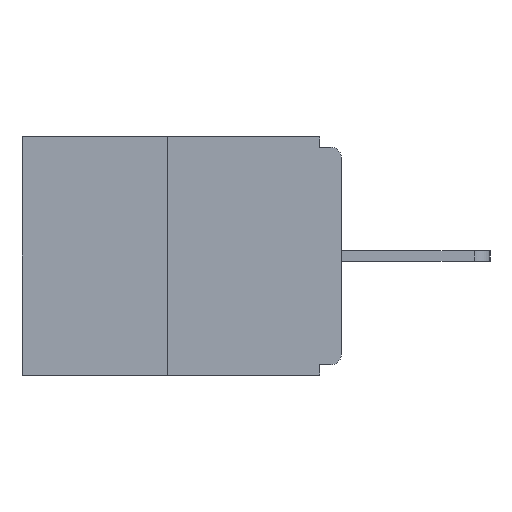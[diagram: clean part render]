
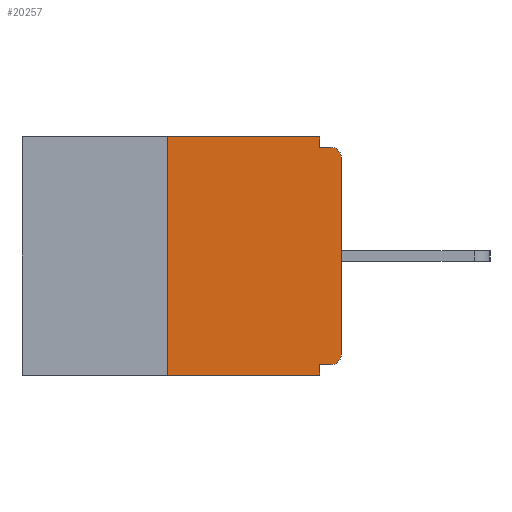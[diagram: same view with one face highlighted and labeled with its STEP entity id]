
A CAD part, left-side view. The second image highlights one B-rep face of the part: STEP entity #20257.
In plain terms, the highlighted planar face has unit normal (-1, 0, 0).
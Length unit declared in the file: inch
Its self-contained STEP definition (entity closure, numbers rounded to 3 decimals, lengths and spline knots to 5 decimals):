
#117 = VECTOR ( 'NONE', #4930, 39.37008 ) ;
#574 = DIRECTION ( 'NONE',  ( 0., -1., 0. ) ) ;
#755 = ORIENTED_EDGE ( 'NONE', *, *, #6911, .F. ) ;
#1035 = VECTOR ( 'NONE', #574, 39.37008 ) ;
#2110 = EDGE_CURVE ( 'NONE', #6179, #14480, #10528, .T. ) ;
#2219 = LINE ( 'NONE', #10563, #1035 ) ;
#2291 = VERTEX_POINT ( 'NONE', #3269 ) ;
#2664 = VERTEX_POINT ( 'NONE', #17698 ) ;
#2714 = CARTESIAN_POINT ( 'NONE',  ( 0., 0.031, 0. ) ) ;
#2983 = ORIENTED_EDGE ( 'NONE', *, *, #8985, .F. ) ;
#3269 = CARTESIAN_POINT ( 'NONE',  ( 0., 0.25, -0.343 ) ) ;
#3301 = ORIENTED_EDGE ( 'NONE', *, *, #9194, .T. ) ;
#3342 = CIRCLE ( 'NONE', #20670, 0.015 ) ;
#3399 = CARTESIAN_POINT ( 'NONE',  ( 0., 0., -0.328 ) ) ;
#3410 = CARTESIAN_POINT ( 'NONE',  ( 0., 0., -0.015 ) ) ;
#3615 = DIRECTION ( 'NONE',  ( 0., 0., 1. ) ) ;
#3663 = VERTEX_POINT ( 'NONE', #17175 ) ;
#3956 = ORIENTED_EDGE ( 'NONE', *, *, #13692, .F. ) ;
#4565 = VECTOR ( 'NONE', #20036, 39.37008 ) ;
#4846 = EDGE_CURVE ( 'NONE', #13878, #9414, #21352, .T. ) ;
#4930 = DIRECTION ( 'NONE',  ( 0., 0., -1. ) ) ;
#4979 = VECTOR ( 'NONE', #15206, 39.37008 ) ;
#5287 = ORIENTED_EDGE ( 'NONE', *, *, #14898, .F. ) ;
#6045 = AXIS2_PLACEMENT_3D ( 'NONE', #9595, #14525, #11502 ) ;
#6106 = VERTEX_POINT ( 'NONE', #14680 ) ;
#6179 = VERTEX_POINT ( 'NONE', #20354 ) ;
#6204 = DIRECTION ( 'NONE',  ( 0., 0., -1. ) ) ;
#6223 = FACE_OUTER_BOUND ( 'NONE', #15611, .T. ) ;
#6728 = LINE ( 'NONE', #12034, #15156 ) ;
#6911 = EDGE_CURVE ( 'NONE', #2664, #8474, #21631, .T. ) ;
#8474 = VERTEX_POINT ( 'NONE', #15916 ) ;
#8921 = CARTESIAN_POINT ( 'NONE',  ( 0., 0.031, -0.015 ) ) ;
#8985 = EDGE_CURVE ( 'NONE', #9414, #6106, #18573, .T. ) ;
#9194 = EDGE_CURVE ( 'NONE', #14480, #6106, #3342, .T. ) ;
#9414 = VERTEX_POINT ( 'NONE', #8921 ) ;
#9595 = CARTESIAN_POINT ( 'NONE',  ( 0., 0.015, -0.313 ) ) ;
#9598 = CIRCLE ( 'NONE', #6045, 0.015 ) ;
#10102 = VECTOR ( 'NONE', #16882, 39.37008 ) ;
#10528 = LINE ( 'NONE', #17203, #20855 ) ;
#10563 = CARTESIAN_POINT ( 'NONE',  ( 0., 0.46, 0. ) ) ;
#11502 = DIRECTION ( 'NONE',  ( 0., 0., -1. ) ) ;
#11679 = CARTESIAN_POINT ( 'NONE',  ( 0., 0., -0.03 ) ) ;
#12034 = CARTESIAN_POINT ( 'NONE',  ( 0., 0.25, 0. ) ) ;
#12941 = PLANE ( 'NONE',  #17561 ) ;
#13042 = EDGE_CURVE ( 'NONE', #2291, #8474, #14574, .T. ) ;
#13259 = CARTESIAN_POINT ( 'NONE',  ( 0., 0.46, -0.343 ) ) ;
#13692 = EDGE_CURVE ( 'NONE', #2291, #17548, #6728, .T. ) ;
#13878 = VERTEX_POINT ( 'NONE', #2714 ) ;
#14049 = ORIENTED_EDGE ( 'NONE', *, *, #20490, .F. ) ;
#14204 = CARTESIAN_POINT ( 'NONE',  ( 0., 0.015, -0.03 ) ) ;
#14217 = VECTOR ( 'NONE', #6204, 39.37008 ) ;
#14480 = VERTEX_POINT ( 'NONE', #11679 ) ;
#14525 = DIRECTION ( 'NONE',  ( -1., 0., 0. ) ) ;
#14574 = LINE ( 'NONE', #13259, #4565 ) ;
#14680 = CARTESIAN_POINT ( 'NONE',  ( 0., 0.015, -0.015 ) ) ;
#14898 = EDGE_CURVE ( 'NONE', #3663, #2664, #18562, .T. ) ;
#15146 = EDGE_CURVE ( 'NONE', #3663, #6179, #9598, .T. ) ;
#15156 = VECTOR ( 'NONE', #3615, 39.37008 ) ;
#15206 = DIRECTION ( 'NONE',  ( 0., 1., 0. ) ) ;
#15210 = DIRECTION ( 'NONE',  ( 0., 0., 1. ) ) ;
#15517 = ORIENTED_EDGE ( 'NONE', *, *, #4846, .F. ) ;
#15611 = EDGE_LOOP ( 'NONE', ( #14049, #3956, #17059, #755, #5287, #18171, #20974, #3301, #2983, #15517 ) ) ;
#15916 = CARTESIAN_POINT ( 'NONE',  ( 0., 0.031, -0.343 ) ) ;
#15958 = DIRECTION ( 'NONE',  ( -1., 0., 0. ) ) ;
#16303 = DIRECTION ( 'NONE',  ( 0., 0., -1. ) ) ;
#16882 = DIRECTION ( 'NONE',  ( 0., -1., 0. ) ) ;
#17059 = ORIENTED_EDGE ( 'NONE', *, *, #13042, .T. ) ;
#17175 = CARTESIAN_POINT ( 'NONE',  ( 0., 0.015, -0.328 ) ) ;
#17203 = CARTESIAN_POINT ( 'NONE',  ( 0., 0., 0. ) ) ;
#17548 = VERTEX_POINT ( 'NONE', #19046 ) ;
#17561 = AXIS2_PLACEMENT_3D ( 'NONE', #19721, #18052, #21806 ) ;
#17698 = CARTESIAN_POINT ( 'NONE',  ( 0., 0.031, -0.328 ) ) ;
#18052 = DIRECTION ( 'NONE',  ( 1., 0., 0. ) ) ;
#18171 = ORIENTED_EDGE ( 'NONE', *, *, #15146, .T. ) ;
#18470 = CARTESIAN_POINT ( 'NONE',  ( 0., 0.031, 0. ) ) ;
#18562 = LINE ( 'NONE', #3399, #4979 ) ;
#18573 = LINE ( 'NONE', #3410, #10102 ) ;
#19046 = CARTESIAN_POINT ( 'NONE',  ( 0., 0.25, 0. ) ) ;
#19721 = CARTESIAN_POINT ( 'NONE',  ( 0., 0.46, 0. ) ) ;
#20036 = DIRECTION ( 'NONE',  ( 0., -1., 0. ) ) ;
#20257 = ADVANCED_FACE ( 'NONE', ( #6223 ), #12941, .F. ) ;
#20354 = CARTESIAN_POINT ( 'NONE',  ( 0., 0., -0.313 ) ) ;
#20490 = EDGE_CURVE ( 'NONE', #17548, #13878, #2219, .T. ) ;
#20670 = AXIS2_PLACEMENT_3D ( 'NONE', #14204, #15958, #16303 ) ;
#20855 = VECTOR ( 'NONE', #15210, 39.37008 ) ;
#20974 = ORIENTED_EDGE ( 'NONE', *, *, #2110, .T. ) ;
#21352 = LINE ( 'NONE', #18470, #14217 ) ;
#21525 = CARTESIAN_POINT ( 'NONE',  ( 0., 0.031, -0.343 ) ) ;
#21631 = LINE ( 'NONE', #21525, #117 ) ;
#21806 = DIRECTION ( 'NONE',  ( 0., 0., -1. ) ) ;
